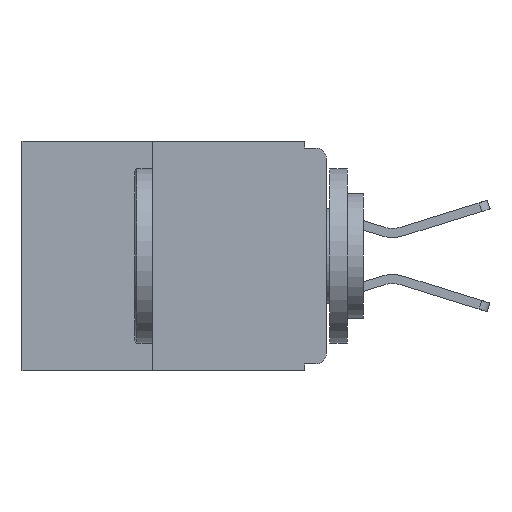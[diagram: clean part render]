
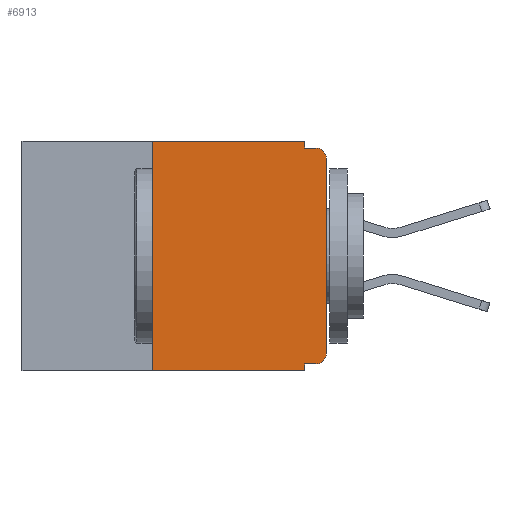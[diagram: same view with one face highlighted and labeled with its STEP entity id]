
A CAD part, left-side view. The second image highlights one B-rep face of the part: STEP entity #6913.
In plain terms, the highlighted planar face has unit normal (-1, 0, 0).
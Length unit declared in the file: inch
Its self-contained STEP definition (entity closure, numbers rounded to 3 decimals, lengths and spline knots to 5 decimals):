
#151 = LINE ( 'NONE', #21812, #12353 ) ;
#963 = DIRECTION ( 'NONE',  ( 0., -1., 0. ) ) ;
#2217 = VERTEX_POINT ( 'NONE', #29689 ) ;
#2515 = VERTEX_POINT ( 'NONE', #9402 ) ;
#2732 = LINE ( 'NONE', #20833, #26996 ) ;
#3511 = DIRECTION ( 'NONE',  ( -1., 0., 0. ) ) ;
#3832 = CARTESIAN_POINT ( 'NONE',  ( 0., 0.031, -0.33 ) ) ;
#4087 = VERTEX_POINT ( 'NONE', #6455 ) ;
#4212 = LINE ( 'NONE', #25888, #21601 ) ;
#4221 = ORIENTED_EDGE ( 'NONE', *, *, #26595, .F. ) ;
#4285 = CARTESIAN_POINT ( 'NONE',  ( 0., 0.015, -0.025 ) ) ;
#4966 = EDGE_CURVE ( 'NONE', #2515, #2217, #17592, .T. ) ;
#5172 = EDGE_LOOP ( 'NONE', ( #29821, #15119, #29485, #13290, #4221, #6632, #8156, #27682, #10684, #23089 ) ) ;
#6455 = CARTESIAN_POINT ( 'NONE',  ( 0., 0.015, -0.01 ) ) ;
#6632 = ORIENTED_EDGE ( 'NONE', *, *, #13055, .F. ) ;
#6774 = DIRECTION ( 'NONE',  ( 0., 0., -1. ) ) ;
#6787 = DIRECTION ( 'NONE',  ( 0., 0., -1. ) ) ;
#6913 = ADVANCED_FACE ( 'NONE', ( #7545 ), #21943, .F. ) ;
#6982 = EDGE_CURVE ( 'NONE', #2217, #24820, #151, .T. ) ;
#7545 = FACE_OUTER_BOUND ( 'NONE', #5172, .T. ) ;
#7766 = LINE ( 'NONE', #14755, #14785 ) ;
#7935 = CARTESIAN_POINT ( 'NONE',  ( 0., 0.031, 0. ) ) ;
#8156 = ORIENTED_EDGE ( 'NONE', *, *, #22063, .T. ) ;
#8424 = CARTESIAN_POINT ( 'NONE',  ( 0., 0.437, -0.33 ) ) ;
#9249 = VERTEX_POINT ( 'NONE', #28076 ) ;
#9402 = CARTESIAN_POINT ( 'NONE',  ( 0., 0.015, -0.32 ) ) ;
#10416 = LINE ( 'NONE', #8424, #22829 ) ;
#10684 = ORIENTED_EDGE ( 'NONE', *, *, #4966, .F. ) ;
#12007 = DIRECTION ( 'NONE',  ( 0., -1., 0. ) ) ;
#12353 = VECTOR ( 'NONE', #21380, 39.37008 ) ;
#12512 = CARTESIAN_POINT ( 'NONE',  ( 0., 0., 0. ) ) ;
#13055 = EDGE_CURVE ( 'NONE', #13936, #28113, #15895, .T. ) ;
#13290 = ORIENTED_EDGE ( 'NONE', *, *, #26936, .F. ) ;
#13936 = VERTEX_POINT ( 'NONE', #17917 ) ;
#14069 = DIRECTION ( 'NONE',  ( 0., 0., 1. ) ) ;
#14092 = VECTOR ( 'NONE', #14873, 39.37008 ) ;
#14755 = CARTESIAN_POINT ( 'NONE',  ( 0., 0.437, 0. ) ) ;
#14785 = VECTOR ( 'NONE', #28531, 39.37008 ) ;
#14873 = DIRECTION ( 'NONE',  ( 0., 0., 1. ) ) ;
#15119 = ORIENTED_EDGE ( 'NONE', *, *, #21060, .T. ) ;
#15415 = VECTOR ( 'NONE', #21262, 39.37008 ) ;
#15692 = VERTEX_POINT ( 'NONE', #7935 ) ;
#15799 = EDGE_CURVE ( 'NONE', #2515, #9249, #27233, .T. ) ;
#15895 = LINE ( 'NONE', #27858, #27396 ) ;
#17323 = AXIS2_PLACEMENT_3D ( 'NONE', #17788, #3511, #20145 ) ;
#17432 = VERTEX_POINT ( 'NONE', #26333 ) ;
#17592 = LINE ( 'NONE', #21556, #15415 ) ;
#17788 = CARTESIAN_POINT ( 'NONE',  ( 0., 0.015, -0.305 ) ) ;
#17906 = EDGE_CURVE ( 'NONE', #23762, #4087, #4212, .T. ) ;
#17917 = CARTESIAN_POINT ( 'NONE',  ( 0., 0.25, -0.33 ) ) ;
#18176 = CIRCLE ( 'NONE', #19380, 0.015 ) ;
#18232 = CARTESIAN_POINT ( 'NONE',  ( 0., 0.25, 0. ) ) ;
#19380 = AXIS2_PLACEMENT_3D ( 'NONE', #4285, #20843, #6787 ) ;
#20145 = DIRECTION ( 'NONE',  ( 0., 0., -1. ) ) ;
#20833 = CARTESIAN_POINT ( 'NONE',  ( 0., 0.031, 0. ) ) ;
#20843 = DIRECTION ( 'NONE',  ( -1., 0., 0. ) ) ;
#21060 = EDGE_CURVE ( 'NONE', #17432, #4087, #18176, .T. ) ;
#21262 = DIRECTION ( 'NONE',  ( 0., 1., 0. ) ) ;
#21380 = DIRECTION ( 'NONE',  ( 0., 0., -1. ) ) ;
#21556 = CARTESIAN_POINT ( 'NONE',  ( 0., 0., -0.32 ) ) ;
#21601 = VECTOR ( 'NONE', #12007, 39.37008 ) ;
#21812 = CARTESIAN_POINT ( 'NONE',  ( 0., 0.031, -0.33 ) ) ;
#21890 = DIRECTION ( 'NONE',  ( 0., 0., -1. ) ) ;
#21911 = DIRECTION ( 'NONE',  ( 1., 0., 0. ) ) ;
#21943 = PLANE ( 'NONE',  #22198 ) ;
#22063 = EDGE_CURVE ( 'NONE', #13936, #24820, #10416, .T. ) ;
#22187 = CARTESIAN_POINT ( 'NONE',  ( 0., 0.437, 0. ) ) ;
#22198 = AXIS2_PLACEMENT_3D ( 'NONE', #22187, #21911, #21890 ) ;
#22829 = VECTOR ( 'NONE', #963, 39.37008 ) ;
#23089 = ORIENTED_EDGE ( 'NONE', *, *, #15799, .T. ) ;
#23762 = VERTEX_POINT ( 'NONE', #25382 ) ;
#24820 = VERTEX_POINT ( 'NONE', #3832 ) ;
#25382 = CARTESIAN_POINT ( 'NONE',  ( 0., 0.031, -0.01 ) ) ;
#25668 = LINE ( 'NONE', #12512, #14092 ) ;
#25729 = EDGE_CURVE ( 'NONE', #9249, #17432, #25668, .T. ) ;
#25888 = CARTESIAN_POINT ( 'NONE',  ( 0., 0., -0.01 ) ) ;
#26333 = CARTESIAN_POINT ( 'NONE',  ( 0., 0., -0.025 ) ) ;
#26595 = EDGE_CURVE ( 'NONE', #28113, #15692, #7766, .T. ) ;
#26936 = EDGE_CURVE ( 'NONE', #15692, #23762, #2732, .T. ) ;
#26996 = VECTOR ( 'NONE', #6774, 39.37008 ) ;
#27233 = CIRCLE ( 'NONE', #17323, 0.015 ) ;
#27396 = VECTOR ( 'NONE', #14069, 39.37008 ) ;
#27682 = ORIENTED_EDGE ( 'NONE', *, *, #6982, .F. ) ;
#27858 = CARTESIAN_POINT ( 'NONE',  ( 0., 0.25, -0.33 ) ) ;
#28076 = CARTESIAN_POINT ( 'NONE',  ( 0., 0., -0.305 ) ) ;
#28113 = VERTEX_POINT ( 'NONE', #18232 ) ;
#28531 = DIRECTION ( 'NONE',  ( 0., -1., 0. ) ) ;
#29485 = ORIENTED_EDGE ( 'NONE', *, *, #17906, .F. ) ;
#29689 = CARTESIAN_POINT ( 'NONE',  ( 0., 0.031, -0.32 ) ) ;
#29821 = ORIENTED_EDGE ( 'NONE', *, *, #25729, .T. ) ;
